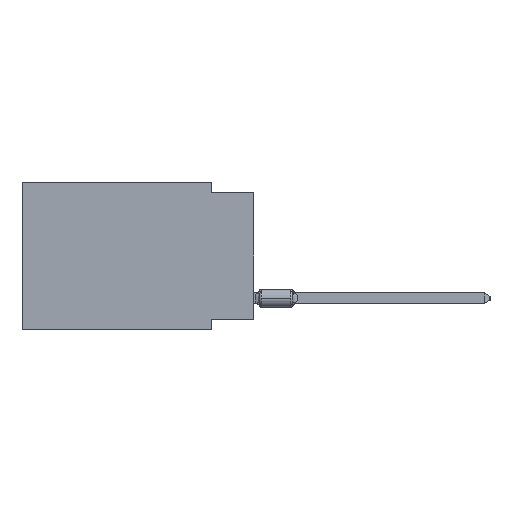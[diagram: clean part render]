
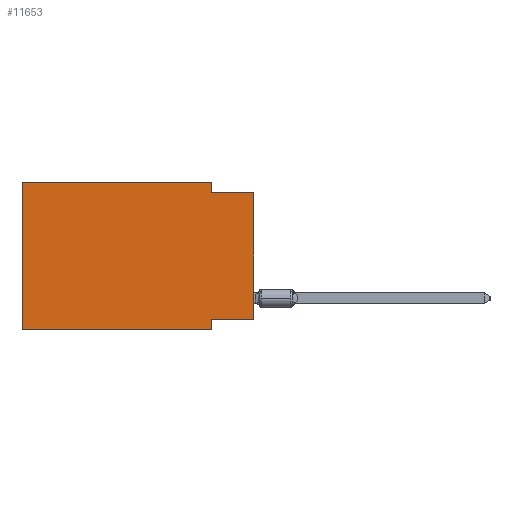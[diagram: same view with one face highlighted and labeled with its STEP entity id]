
A CAD part, left-side view. The second image highlights one B-rep face of the part: STEP entity #11653.
In plain terms, the highlighted planar face has unit normal (-1, 0, 0).
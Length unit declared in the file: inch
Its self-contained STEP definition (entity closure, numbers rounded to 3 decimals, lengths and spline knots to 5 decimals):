
#179 = CARTESIAN_POINT ( 'NONE',  ( 0., 0.55, -0.35 ) ) ;
#620 = VERTEX_POINT ( 'NONE', #15823 ) ;
#956 = VERTEX_POINT ( 'NONE', #23808 ) ;
#2050 = CARTESIAN_POINT ( 'NONE',  ( 0., 0., -0.025 ) ) ;
#3534 = DIRECTION ( 'NONE',  ( 0., 1., 0. ) ) ;
#4479 = CARTESIAN_POINT ( 'NONE',  ( 0., 0.55, 0. ) ) ;
#5335 = EDGE_CURVE ( 'NONE', #24109, #31832, #27883, .T. ) ;
#5843 = EDGE_CURVE ( 'NONE', #620, #6812, #11453, .T. ) ;
#6096 = PLANE ( 'NONE',  #33933 ) ;
#6812 = VERTEX_POINT ( 'NONE', #2050 ) ;
#7852 = VERTEX_POINT ( 'NONE', #13377 ) ;
#7880 = LINE ( 'NONE', #26016, #18264 ) ;
#8115 = LINE ( 'NONE', #32193, #11132 ) ;
#10217 = DIRECTION ( 'NONE',  ( 0., 0., 1. ) ) ;
#10269 = CARTESIAN_POINT ( 'NONE',  ( 0., 0.1, 0. ) ) ;
#10336 = CARTESIAN_POINT ( 'NONE',  ( 0., 0.55, 0. ) ) ;
#11132 = VECTOR ( 'NONE', #18406, 39.37008 ) ;
#11335 = LINE ( 'NONE', #179, #27705 ) ;
#11453 = LINE ( 'NONE', #19943, #23754 ) ;
#11653 = ADVANCED_FACE ( 'NONE', ( #28050 ), #6096, .F. ) ;
#12252 = EDGE_CURVE ( 'NONE', #956, #6812, #15558, .T. ) ;
#12347 = VECTOR ( 'NONE', #10217, 39.37008 ) ;
#12611 = CARTESIAN_POINT ( 'NONE',  ( 0., 0., 0. ) ) ;
#13377 = CARTESIAN_POINT ( 'NONE',  ( 0., 0.1, -0.35 ) ) ;
#13560 = EDGE_CURVE ( 'NONE', #26836, #7852, #8115, .T. ) ;
#14069 = ORIENTED_EDGE ( 'NONE', *, *, #16749, .F. ) ;
#14101 = DIRECTION ( 'NONE',  ( 0., -1., 0. ) ) ;
#14273 = DIRECTION ( 'NONE',  ( 1., 0., 0. ) ) ;
#15030 = ORIENTED_EDGE ( 'NONE', *, *, #5335, .F. ) ;
#15222 = DIRECTION ( 'NONE',  ( 0., -1., 0. ) ) ;
#15383 = DIRECTION ( 'NONE',  ( 0., 0., 1. ) ) ;
#15558 = LINE ( 'NONE', #12611, #21058 ) ;
#15823 = CARTESIAN_POINT ( 'NONE',  ( 0., 0.1, -0.025 ) ) ;
#16233 = DIRECTION ( 'NONE',  ( 0., -1., 0. ) ) ;
#16323 = ORIENTED_EDGE ( 'NONE', *, *, #32585, .F. ) ;
#16749 = EDGE_CURVE ( 'NONE', #34127, #24109, #17909, .T. ) ;
#17909 = LINE ( 'NONE', #4479, #12347 ) ;
#18264 = VECTOR ( 'NONE', #20936, 39.37008 ) ;
#18406 = DIRECTION ( 'NONE',  ( 0., 0., -1. ) ) ;
#18963 = CARTESIAN_POINT ( 'NONE',  ( 0., 0.1, -0.325 ) ) ;
#19229 = ORIENTED_EDGE ( 'NONE', *, *, #13560, .F. ) ;
#19517 = DIRECTION ( 'NONE',  ( 0., 0., -1. ) ) ;
#19943 = CARTESIAN_POINT ( 'NONE',  ( 0., 0., -0.025 ) ) ;
#20936 = DIRECTION ( 'NONE',  ( 0., 0., -1. ) ) ;
#21058 = VECTOR ( 'NONE', #15383, 39.37008 ) ;
#21674 = LINE ( 'NONE', #27264, #22071 ) ;
#21842 = EDGE_LOOP ( 'NONE', ( #26088, #31880, #16323, #15030, #14069, #33226, #19229, #30503 ) ) ;
#22071 = VECTOR ( 'NONE', #3534, 39.37008 ) ;
#22294 = CARTESIAN_POINT ( 'NONE',  ( 0., 0.55, 0. ) ) ;
#23676 = CARTESIAN_POINT ( 'NONE',  ( 0., 0.55, -0.35 ) ) ;
#23754 = VECTOR ( 'NONE', #15222, 39.37008 ) ;
#23808 = CARTESIAN_POINT ( 'NONE',  ( 0., 0., -0.325 ) ) ;
#24109 = VERTEX_POINT ( 'NONE', #10336 ) ;
#24629 = EDGE_CURVE ( 'NONE', #34127, #7852, #11335, .T. ) ;
#26016 = CARTESIAN_POINT ( 'NONE',  ( 0., 0.1, 0. ) ) ;
#26088 = ORIENTED_EDGE ( 'NONE', *, *, #12252, .T. ) ;
#26836 = VERTEX_POINT ( 'NONE', #18963 ) ;
#27264 = CARTESIAN_POINT ( 'NONE',  ( 0., 0., -0.325 ) ) ;
#27705 = VECTOR ( 'NONE', #16233, 39.37008 ) ;
#27883 = LINE ( 'NONE', #22294, #29717 ) ;
#28050 = FACE_OUTER_BOUND ( 'NONE', #21842, .T. ) ;
#29717 = VECTOR ( 'NONE', #14101, 39.37008 ) ;
#30229 = EDGE_CURVE ( 'NONE', #956, #26836, #21674, .T. ) ;
#30324 = CARTESIAN_POINT ( 'NONE',  ( 0., 0.55, 0. ) ) ;
#30503 = ORIENTED_EDGE ( 'NONE', *, *, #30229, .F. ) ;
#31832 = VERTEX_POINT ( 'NONE', #10269 ) ;
#31880 = ORIENTED_EDGE ( 'NONE', *, *, #5843, .F. ) ;
#32193 = CARTESIAN_POINT ( 'NONE',  ( 0., 0.1, -0.35 ) ) ;
#32585 = EDGE_CURVE ( 'NONE', #31832, #620, #7880, .T. ) ;
#33226 = ORIENTED_EDGE ( 'NONE', *, *, #24629, .T. ) ;
#33933 = AXIS2_PLACEMENT_3D ( 'NONE', #30324, #14273, #19517 ) ;
#34127 = VERTEX_POINT ( 'NONE', #23676 ) ;
